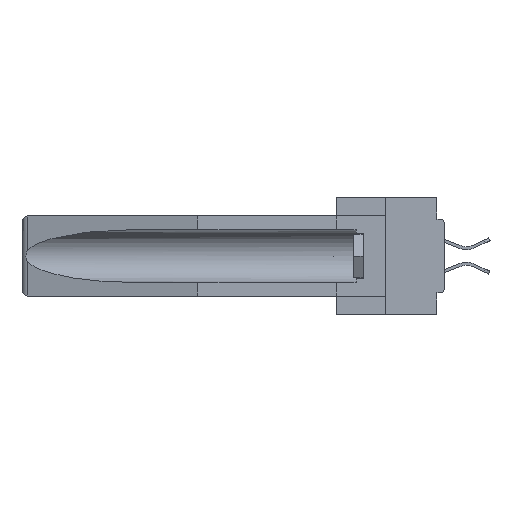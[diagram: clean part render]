
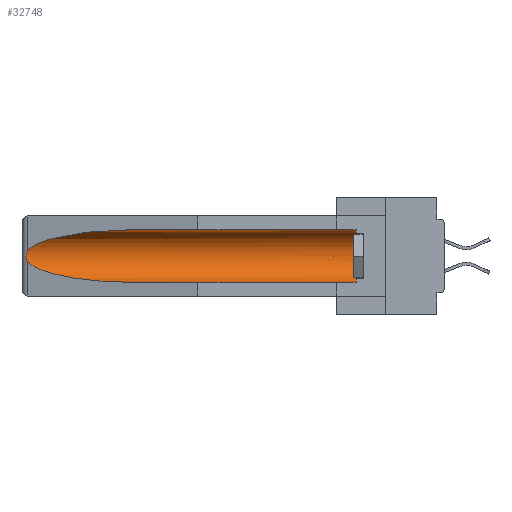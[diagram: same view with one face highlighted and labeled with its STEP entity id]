
A CAD part, left-side view. The second image highlights one B-rep face of the part: STEP entity #32748.
In plain terms, the highlighted cylindrical face has radius 2.857 mm (diameter 5.715 mm), a partial arc.
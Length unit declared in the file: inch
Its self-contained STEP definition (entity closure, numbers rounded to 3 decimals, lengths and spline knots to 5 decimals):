
#338 = EDGE_CURVE ( 'NONE', #24689, #9938, #40287, .T. ) ;
#1301 = ORIENTED_EDGE ( 'NONE', *, *, #338, .T. ) ;
#1887 = EDGE_CURVE ( 'NONE', #15440, #40846, #4483, .T. ) ;
#2340 = CARTESIAN_POINT ( 'NONE',  ( 0.2673, 1.53269, -0.17917 ) ) ;
#3036 = VERTEX_POINT ( 'NONE', #16278 ) ;
#3175 = LINE ( 'NONE', #21650, #5502 ) ;
#4483 = CIRCLE ( 'NONE', #46054, 0.1125 ) ;
#5141 = CARTESIAN_POINT ( 'NONE',  ( 0.26537, 1.52718, -0.19328 ) ) ;
#5502 = VECTOR ( 'NONE', #36770, 39.37008 ) ;
#5873 = EDGE_CURVE ( 'NONE', #15440, #3036, #3175, .T. ) ;
#6550 = ORIENTED_EDGE ( 'NONE', *, *, #5873, .F. ) ;
#6741 = DIRECTION ( 'NONE',  ( 0., 0., 1. ) ) ;
#7762 = ORIENTED_EDGE ( 'NONE', *, *, #39279, .T. ) ;
#7839 = CARTESIAN_POINT ( 'NONE',  ( 0.26537, 1.52718, -0.14972 ) ) ;
#9634 = CARTESIAN_POINT ( 'NONE',  ( 0.26597, 1.52961, -0.15275 ) ) ;
#9796 = CARTESIAN_POINT ( 'NONE',  ( 0.2675, 1.53308, -0.16763 ) ) ;
#9938 = VERTEX_POINT ( 'NONE', #7839 ) ;
#10153 = DIRECTION ( 'NONE',  ( 0., -1., 0. ) ) ;
#10266 = CARTESIAN_POINT ( 'NONE',  ( 0.2675, 1.53308, -0.17534 ) ) ;
#10832 = B_SPLINE_CURVE_WITH_KNOTS ( 'NONE', 3,
 ( #25017, #9634, #32516, #17256, #9796, #10266, #2340, #35786, #28580, #24537 ),
 .UNSPECIFIED., .F., .F.,
 ( 4, 2, 2, 2, 4 ),
 ( 0., 0.00029, 0.00058, 0.00087, 0.00117 ),
 .UNSPECIFIED. ) ;
#12816 = FACE_OUTER_BOUND ( 'NONE', #41790, .T. ) ;
#15057 = CARTESIAN_POINT ( 'NONE',  ( 0.26537, 1.52718, -0.19328 ) ) ;
#15440 = VERTEX_POINT ( 'NONE', #35477 ) ;
#16278 = CARTESIAN_POINT ( 'NONE',  ( 0.155, 1.07973, -0.284 ) ) ;
#16841 = ORIENTED_EDGE ( 'NONE', *, *, #29560, .T. ) ;
#16848 = DIRECTION ( 'NONE',  ( 0., 0., 1. ) ) ;
#17223 = CARTESIAN_POINT ( 'NONE',  ( 0.155, -0.30754, -0.059 ) ) ;
#17256 = CARTESIAN_POINT ( 'NONE',  ( 0.2673, 1.5327, -0.16383 ) ) ;
#17412 = EDGE_CURVE ( 'NONE', #9938, #45272, #10832, .T. ) ;
#17483 = CYLINDRICAL_SURFACE ( 'NONE', #45957, 0.1125 ) ;
#20580 = DIRECTION ( 'NONE',  ( 0., 1., 0. ) ) ;
#21650 = CARTESIAN_POINT ( 'NONE',  ( 0.155, -0.30754, -0.284 ) ) ;
#21681 = VECTOR ( 'NONE', #20580, 39.37008 ) ;
#23981 = DIRECTION ( 'NONE',  ( 0., 1., 0. ) ) ;
#24011 = CARTESIAN_POINT ( 'NONE',  ( 0.155, 0.126, -0.059 ) ) ;
#24537 = CARTESIAN_POINT ( 'NONE',  ( 0.26537, 1.52718, -0.19328 ) ) ;
#24689 = VERTEX_POINT ( 'NONE', #34783 ) ;
#25017 = CARTESIAN_POINT ( 'NONE',  ( 0.26537, 1.52718, -0.14972 ) ) ;
#25759 = ORIENTED_EDGE ( 'NONE', *, *, #17412, .T. ) ;
#26959 = ORIENTED_EDGE ( 'NONE', *, *, #1887, .T. ) ;
#28580 = CARTESIAN_POINT ( 'NONE',  ( 0.26597, 1.5296, -0.19026 ) ) ;
#29560 = EDGE_CURVE ( 'NONE', #45272, #3036, #44698, .T. ) ;
#30300 = CARTESIAN_POINT ( 'NONE',  ( 0.25451, 1.48313, -0.09465 ) ) ;
#31055 = CARTESIAN_POINT ( 'NONE',  ( 0.21114, 1.30732, -0.284 ) ) ;
#31560 = LINE ( 'NONE', #17223, #21681 ) ;
#32516 = CARTESIAN_POINT ( 'NONE',  ( 0.26654, 1.53092, -0.15636 ) ) ;
#32748 = ADVANCED_FACE ( 'NONE', ( #12816 ), #17483, .F. ) ;
#34783 = CARTESIAN_POINT ( 'NONE',  ( 0.155, 1.07973, -0.059 ) ) ;
#35180 = CARTESIAN_POINT ( 'NONE',  ( 0.155, 1.07973, -0.284 ) ) ;
#35477 = CARTESIAN_POINT ( 'NONE',  ( 0.155, 0.126, -0.284 ) ) ;
#35786 = CARTESIAN_POINT ( 'NONE',  ( 0.26655, 1.53094, -0.18657 ) ) ;
#36770 = DIRECTION ( 'NONE',  ( 0., 1., 0. ) ) ;
#37673 = CARTESIAN_POINT ( 'NONE',  ( 0.155, 1.07973, -0.059 ) ) ;
#39133 = CARTESIAN_POINT ( 'NONE',  ( 0.155, -0.30754, -0.1715 ) ) ;
#39279 = EDGE_CURVE ( 'NONE', #40846, #24689, #31560, .T. ) ;
#40287 =( BOUNDED_CURVE ( )  B_SPLINE_CURVE ( 3, ( #37673, #41397, #30300, #44636 ),
 .UNSPECIFIED., .F., .F. ) 
 B_SPLINE_CURVE_WITH_KNOTS ( ( 4, 4 ),
 ( 4.71239, 6.08839 ),
 .UNSPECIFIED. ) 
 CURVE ( )  GEOMETRIC_REPRESENTATION_ITEM ( )  RATIONAL_B_SPLINE_CURVE ( ( 1., 0.848, 0.848, 1. ) ) 
 REPRESENTATION_ITEM ( '' )  );
#40846 = VERTEX_POINT ( 'NONE', #24011 ) ;
#41397 = CARTESIAN_POINT ( 'NONE',  ( 0.21114, 1.30732, -0.059 ) ) ;
#41790 = EDGE_LOOP ( 'NONE', ( #1301, #25759, #16841, #6550, #26959, #7762 ) ) ;
#44636 = CARTESIAN_POINT ( 'NONE',  ( 0.26537, 1.52718, -0.14972 ) ) ;
#44698 =( BOUNDED_CURVE ( )  B_SPLINE_CURVE ( 3, ( #5141, #45864, #31055, #35180 ),
 .UNSPECIFIED., .F., .F. ) 
 B_SPLINE_CURVE_WITH_KNOTS ( ( 4, 4 ),
 ( 0.1948, 1.5708 ),
 .UNSPECIFIED. ) 
 CURVE ( )  GEOMETRIC_REPRESENTATION_ITEM ( )  RATIONAL_B_SPLINE_CURVE ( ( 1., 0.848, 0.848, 1. ) ) 
 REPRESENTATION_ITEM ( '' )  );
#45272 = VERTEX_POINT ( 'NONE', #15057 ) ;
#45864 = CARTESIAN_POINT ( 'NONE',  ( 0.25451, 1.48313, -0.24835 ) ) ;
#45957 = AXIS2_PLACEMENT_3D ( 'NONE', #39133, #23981, #16848 ) ;
#46054 = AXIS2_PLACEMENT_3D ( 'NONE', #47640, #10153, #6741 ) ;
#47640 = CARTESIAN_POINT ( 'NONE',  ( 0.155, 0.126, -0.1715 ) ) ;
